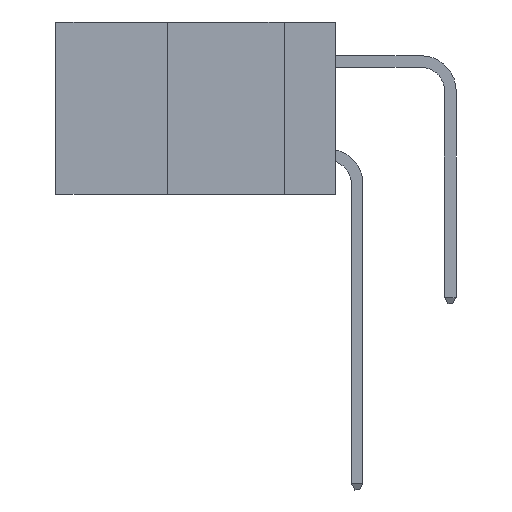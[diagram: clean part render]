
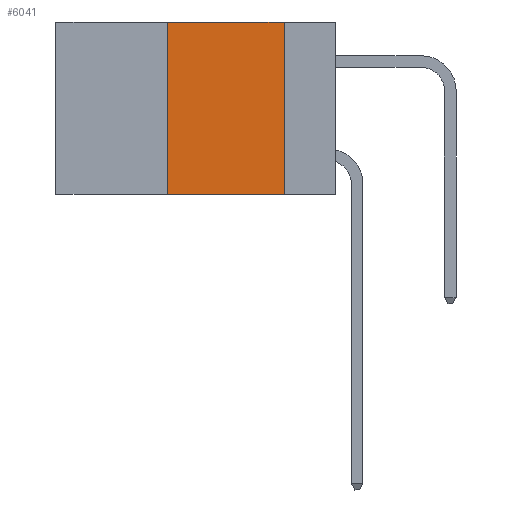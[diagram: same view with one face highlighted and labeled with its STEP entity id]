
A CAD part, left-side view. The second image highlights one B-rep face of the part: STEP entity #6041.
In plain terms, the highlighted planar face has unit normal (-1, 0, 0).
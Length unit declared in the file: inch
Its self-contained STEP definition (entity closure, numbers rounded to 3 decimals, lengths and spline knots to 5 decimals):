
#78 = VERTEX_POINT ( 'NONE', #3953 ) ;
#156 = VERTEX_POINT ( 'NONE', #6516 ) ;
#422 = ORIENTED_EDGE ( 'NONE', *, *, #6895, .F. ) ;
#501 = ORIENTED_EDGE ( 'NONE', *, *, #3119, .F. ) ;
#517 = ORIENTED_EDGE ( 'NONE', *, *, #9631, .F. ) ;
#534 = VECTOR ( 'NONE', #13098, 39.37008 ) ;
#670 = ORIENTED_EDGE ( 'NONE', *, *, #2986, .T. ) ;
#1188 = CARTESIAN_POINT ( 'NONE',  ( 0., 0.36, 0. ) ) ;
#1595 = DIRECTION ( 'NONE',  ( 1., 0., 0. ) ) ;
#2002 = DIRECTION ( 'NONE',  ( 0., 0., -1. ) ) ;
#2088 = VECTOR ( 'NONE', #4715, 39.37008 ) ;
#2538 = EDGE_LOOP ( 'NONE', ( #422, #501, #517, #670 ) ) ;
#2986 = EDGE_CURVE ( 'NONE', #9445, #13642, #9140, .T. ) ;
#3119 = EDGE_CURVE ( 'NONE', #156, #78, #12712, .T. ) ;
#3953 = CARTESIAN_POINT ( 'NONE',  ( 0., 0.11, 0. ) ) ;
#4715 = DIRECTION ( 'NONE',  ( 0., -1., 0. ) ) ;
#4957 = CARTESIAN_POINT ( 'NONE',  ( 0., 0.6, 0. ) ) ;
#6041 = ADVANCED_FACE ( 'NONE', ( #6990 ), #8718, .F. ) ;
#6516 = CARTESIAN_POINT ( 'NONE',  ( 0., 0.36, 0. ) ) ;
#6895 = EDGE_CURVE ( 'NONE', #78, #13642, #14366, .T. ) ;
#6990 = FACE_OUTER_BOUND ( 'NONE', #2538, .T. ) ;
#7211 = CARTESIAN_POINT ( 'NONE',  ( 0., 0.11, -0.37 ) ) ;
#7913 = CARTESIAN_POINT ( 'NONE',  ( 0., 0.11, 0. ) ) ;
#8324 = DIRECTION ( 'NONE',  ( 0., 0., 1. ) ) ;
#8664 = VECTOR ( 'NONE', #2002, 39.37008 ) ;
#8718 = PLANE ( 'NONE',  #9451 ) ;
#9037 = VECTOR ( 'NONE', #8324, 39.37008 ) ;
#9140 = LINE ( 'NONE', #9367, #2088 ) ;
#9367 = CARTESIAN_POINT ( 'NONE',  ( 0., 0.6, -0.37 ) ) ;
#9445 = VERTEX_POINT ( 'NONE', #13673 ) ;
#9451 = AXIS2_PLACEMENT_3D ( 'NONE', #13232, #1595, #9923 ) ;
#9631 = EDGE_CURVE ( 'NONE', #9445, #156, #12112, .T. ) ;
#9923 = DIRECTION ( 'NONE',  ( 0., 0., -1. ) ) ;
#12112 = LINE ( 'NONE', #1188, #9037 ) ;
#12712 = LINE ( 'NONE', #4957, #534 ) ;
#13098 = DIRECTION ( 'NONE',  ( 0., -1., 0. ) ) ;
#13232 = CARTESIAN_POINT ( 'NONE',  ( 0., 0.6, 0. ) ) ;
#13642 = VERTEX_POINT ( 'NONE', #7211 ) ;
#13673 = CARTESIAN_POINT ( 'NONE',  ( 0., 0.36, -0.37 ) ) ;
#14366 = LINE ( 'NONE', #7913, #8664 ) ;
